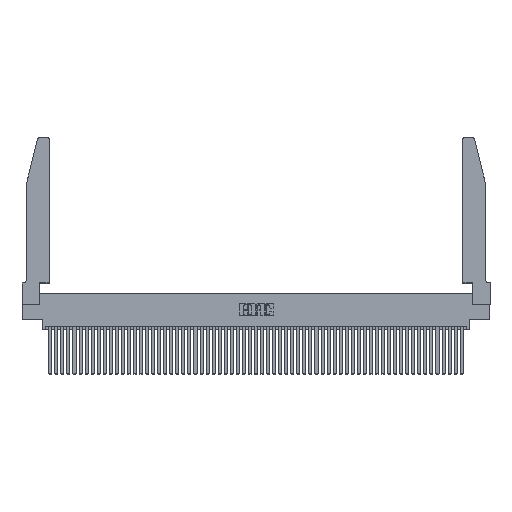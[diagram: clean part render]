
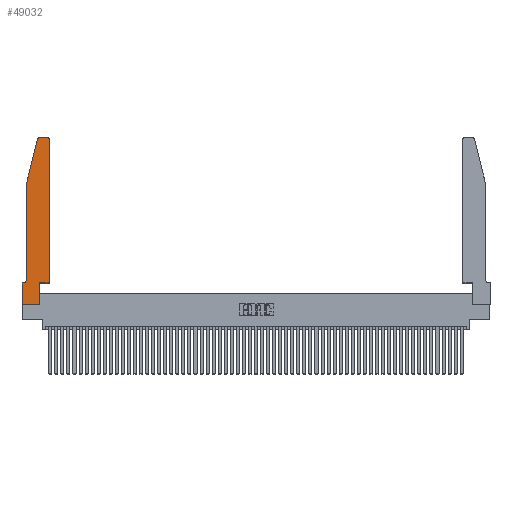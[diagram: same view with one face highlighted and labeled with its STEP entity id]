
A CAD part, top view. The second image highlights one B-rep face of the part: STEP entity #49032.
In plain terms, the highlighted planar face has unit normal (0, 0, 1).
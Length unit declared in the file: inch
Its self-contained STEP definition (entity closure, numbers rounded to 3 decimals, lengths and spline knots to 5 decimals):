
#234 = CARTESIAN_POINT ( 'NONE',  ( 0.0055, 0.35, 0.37 ) ) ;
#356 = PLANE ( 'NONE',  #37514 ) ;
#2362 = LINE ( 'NONE', #2958, #35053 ) ;
#2537 = EDGE_CURVE ( 'NONE', #3211, #25090, #53516, .T. ) ;
#2841 = EDGE_CURVE ( 'NONE', #51673, #12014, #40145, .T. ) ;
#2958 = CARTESIAN_POINT ( 'NONE',  ( 0.0755, 0.35, 0.37 ) ) ;
#3211 = VERTEX_POINT ( 'NONE', #28356 ) ;
#3332 = VECTOR ( 'NONE', #48584, 39.37008 ) ;
#4187 = VECTOR ( 'NONE', #5043, 39.37008 ) ;
#4496 = LINE ( 'NONE', #52020, #51205 ) ;
#4676 = VECTOR ( 'NONE', #13971, 39.37008 ) ;
#4893 = AXIS2_PLACEMENT_3D ( 'NONE', #32284, #6732, #36550 ) ;
#5043 = DIRECTION ( 'NONE',  ( -1., 0., 0. ) ) ;
#6732 = DIRECTION ( 'NONE',  ( 0., 0., -1. ) ) ;
#7258 = DIRECTION ( 'NONE',  ( -1., 0., 0. ) ) ;
#7620 = VERTEX_POINT ( 'NONE', #11409 ) ;
#8999 = DIRECTION ( 'NONE',  ( 0., 0., 1. ) ) ;
#9119 = EDGE_CURVE ( 'NONE', #49681, #10168, #4496, .T. ) ;
#9501 = EDGE_CURVE ( 'NONE', #7620, #22272, #21219, .T. ) ;
#9557 = DIRECTION ( 'NONE',  ( 0., 0., 1. ) ) ;
#10168 = VERTEX_POINT ( 'NONE', #13776 ) ;
#11409 = CARTESIAN_POINT ( 'NONE',  ( 0., 0., 0.37 ) ) ;
#11883 = CARTESIAN_POINT ( 'NONE',  ( 0.284, 2.75, 0.37 ) ) ;
#12014 = VERTEX_POINT ( 'NONE', #50816 ) ;
#12267 = AXIS2_PLACEMENT_3D ( 'NONE', #50193, #24739, #54454 ) ;
#12607 = CARTESIAN_POINT ( 'NONE',  ( 0.0755, 2., 0.37 ) ) ;
#13776 = CARTESIAN_POINT ( 'NONE',  ( 0.4505, 2.72, 0.37 ) ) ;
#13804 = CARTESIAN_POINT ( 'NONE',  ( 0., 0., 0.37 ) ) ;
#13971 = DIRECTION ( 'NONE',  ( 0., -1., 0. ) ) ;
#14745 = LINE ( 'NONE', #23157, #3332 ) ;
#15158 = ORIENTED_EDGE ( 'NONE', *, *, #49406, .T. ) ;
#15579 = LINE ( 'NONE', #39156, #4187 ) ;
#16317 = EDGE_CURVE ( 'NONE', #28618, #49681, #23749, .T. ) ;
#16834 = CARTESIAN_POINT ( 'NONE',  ( 0.0755, 2., 0.37 ) ) ;
#17125 = ORIENTED_EDGE ( 'NONE', *, *, #51018, .T. ) ;
#17288 = VERTEX_POINT ( 'NONE', #11883 ) ;
#17553 = VECTOR ( 'NONE', #21142, 39.37008 ) ;
#17594 = VERTEX_POINT ( 'NONE', #30838 ) ;
#21142 = DIRECTION ( 'NONE',  ( -0.239, -0.971, 0. ) ) ;
#21161 = ORIENTED_EDGE ( 'NONE', *, *, #2841, .T. ) ;
#21170 = FACE_OUTER_BOUND ( 'NONE', #34915, .T. ) ;
#21219 = LINE ( 'NONE', #47148, #53805 ) ;
#21418 = EDGE_CURVE ( 'NONE', #22272, #28618, #14745, .T. ) ;
#21869 = ORIENTED_EDGE ( 'NONE', *, *, #9501, .T. ) ;
#22272 = VERTEX_POINT ( 'NONE', #23995 ) ;
#22409 = VECTOR ( 'NONE', #30759, 39.37008 ) ;
#22508 = ORIENTED_EDGE ( 'NONE', *, *, #2537, .T. ) ;
#23019 = CIRCLE ( 'NONE', #26969, 0.03 ) ;
#23157 = CARTESIAN_POINT ( 'NONE',  ( 0.2865, 0.35, 0.37 ) ) ;
#23749 = LINE ( 'NONE', #35008, #22409 ) ;
#23995 = CARTESIAN_POINT ( 'NONE',  ( 0.2865, 0., 0.37 ) ) ;
#24739 = DIRECTION ( 'NONE',  ( 0., 0., 1. ) ) ;
#25090 = VERTEX_POINT ( 'NONE', #234 ) ;
#25868 = ORIENTED_EDGE ( 'NONE', *, *, #16317, .T. ) ;
#25957 = DIRECTION ( 'NONE',  ( 1., 0., 0. ) ) ;
#26536 = DIRECTION ( 'NONE',  ( 0., 1., 0. ) ) ;
#26969 = AXIS2_PLACEMENT_3D ( 'NONE', #35057, #9557, #39329 ) ;
#28319 = EDGE_CURVE ( 'NONE', #17288, #51673, #23019, .T. ) ;
#28356 = CARTESIAN_POINT ( 'NONE',  ( 0.0755, 0.42, 0.37 ) ) ;
#28618 = VERTEX_POINT ( 'NONE', #32618 ) ;
#29840 = ORIENTED_EDGE ( 'NONE', *, *, #50707, .T. ) ;
#30010 = CARTESIAN_POINT ( 'NONE',  ( 0.4505, 0.35, 0.37 ) ) ;
#30759 = DIRECTION ( 'NONE',  ( 1., 0., 0. ) ) ;
#30838 = CARTESIAN_POINT ( 'NONE',  ( 0.4205, 2.75, 0.37 ) ) ;
#32284 = CARTESIAN_POINT ( 'NONE',  ( 0.0055, 0.42, 0.37 ) ) ;
#32618 = CARTESIAN_POINT ( 'NONE',  ( 0.2865, 0.35, 0.37 ) ) ;
#34506 = CARTESIAN_POINT ( 'NONE',  ( 0., 0.35, 0.37 ) ) ;
#34915 = EDGE_LOOP ( 'NONE', ( #17125, #51088, #21161, #55073, #22508, #15158, #49108, #21869, #47150, #25868, #48467, #29840 ) ) ;
#35008 = CARTESIAN_POINT ( 'NONE',  ( 0.4505, 0.35, 0.37 ) ) ;
#35053 = VECTOR ( 'NONE', #7258, 39.37008 ) ;
#35057 = CARTESIAN_POINT ( 'NONE',  ( 0.284, 2.72, 0.37 ) ) ;
#36550 = DIRECTION ( 'NONE',  ( -1., 0., 0. ) ) ;
#36638 = VECTOR ( 'NONE', #42332, 39.37008 ) ;
#37514 = AXIS2_PLACEMENT_3D ( 'NONE', #34506, #8999, #38790 ) ;
#38712 = LINE ( 'NONE', #13804, #4676 ) ;
#38790 = DIRECTION ( 'NONE',  ( 1., 0., 0. ) ) ;
#38945 = VERTEX_POINT ( 'NONE', #49795 ) ;
#39156 = CARTESIAN_POINT ( 'NONE',  ( 0.2605, 2.75, 0.37 ) ) ;
#39329 = DIRECTION ( 'NONE',  ( 1., 0., 0. ) ) ;
#40145 = LINE ( 'NONE', #16834, #17553 ) ;
#40632 = LINE ( 'NONE', #12607, #36638 ) ;
#42332 = DIRECTION ( 'NONE',  ( 0., -1., 0. ) ) ;
#44249 = CIRCLE ( 'NONE', #12267, 0.03 ) ;
#46418 = EDGE_CURVE ( 'NONE', #12014, #3211, #40632, .T. ) ;
#47148 = CARTESIAN_POINT ( 'NONE',  ( 0., 0., 0.37 ) ) ;
#47150 = ORIENTED_EDGE ( 'NONE', *, *, #21418, .T. ) ;
#48467 = ORIENTED_EDGE ( 'NONE', *, *, #9119, .T. ) ;
#48584 = DIRECTION ( 'NONE',  ( 0., 1., 0. ) ) ;
#49032 = ADVANCED_FACE ( 'NONE', ( #21170 ), #356, .T. ) ;
#49108 = ORIENTED_EDGE ( 'NONE', *, *, #54603, .T. ) ;
#49406 = EDGE_CURVE ( 'NONE', #25090, #38945, #2362, .T. ) ;
#49681 = VERTEX_POINT ( 'NONE', #30010 ) ;
#49795 = CARTESIAN_POINT ( 'NONE',  ( 0., 0.35, 0.37 ) ) ;
#50193 = CARTESIAN_POINT ( 'NONE',  ( 0.4205, 2.72, 0.37 ) ) ;
#50595 = CARTESIAN_POINT ( 'NONE',  ( 0.25487, 2.72718, 0.37 ) ) ;
#50707 = EDGE_CURVE ( 'NONE', #10168, #17594, #44249, .T. ) ;
#50816 = CARTESIAN_POINT ( 'NONE',  ( 0.0755, 2., 0.37 ) ) ;
#51018 = EDGE_CURVE ( 'NONE', #17594, #17288, #15579, .T. ) ;
#51088 = ORIENTED_EDGE ( 'NONE', *, *, #28319, .T. ) ;
#51205 = VECTOR ( 'NONE', #26536, 39.37008 ) ;
#51673 = VERTEX_POINT ( 'NONE', #50595 ) ;
#52020 = CARTESIAN_POINT ( 'NONE',  ( 0.4505, 0.35, 0.37 ) ) ;
#53516 = CIRCLE ( 'NONE', #4893, 0.07 ) ;
#53805 = VECTOR ( 'NONE', #25957, 39.37008 ) ;
#54454 = DIRECTION ( 'NONE',  ( 1., 0., 0. ) ) ;
#54603 = EDGE_CURVE ( 'NONE', #38945, #7620, #38712, .T. ) ;
#55073 = ORIENTED_EDGE ( 'NONE', *, *, #46418, .T. ) ;
